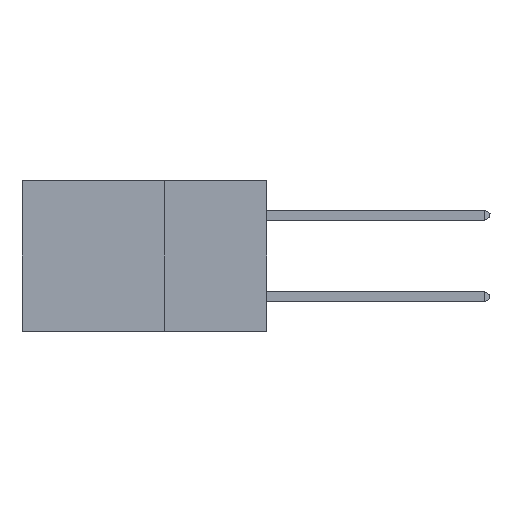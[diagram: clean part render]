
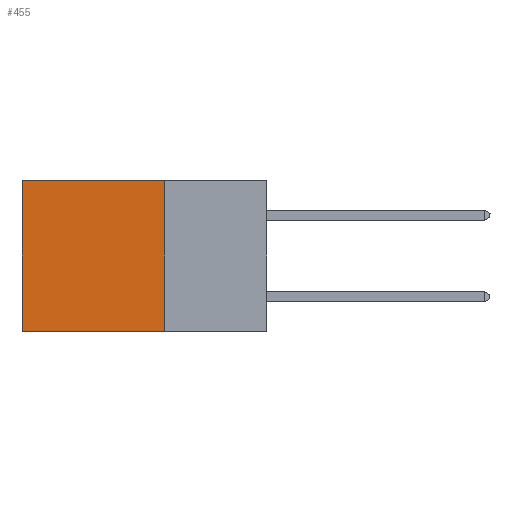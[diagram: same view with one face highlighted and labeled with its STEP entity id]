
A CAD part, left-side view. The second image highlights one B-rep face of the part: STEP entity #455.
In plain terms, the highlighted planar face has unit normal (-1, 0, 0).
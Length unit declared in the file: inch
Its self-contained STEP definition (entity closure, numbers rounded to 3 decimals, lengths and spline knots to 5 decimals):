
#174 = AXIS2_PLACEMENT_3D ( 'NONE', #11066, #1881, #10893 ) ;
#455 = ADVANCED_FACE ( 'NONE', ( #9174 ), #5852, .F. ) ;
#1270 = ORIENTED_EDGE ( 'NONE', *, *, #15241, .T. ) ;
#1368 = ORIENTED_EDGE ( 'NONE', *, *, #4803, .F. ) ;
#1848 = CARTESIAN_POINT ( 'NONE',  ( 0.2875, 0.25, 0. ) ) ;
#1881 = DIRECTION ( 'NONE',  ( 1., 0., 0. ) ) ;
#2020 = VERTEX_POINT ( 'NONE', #3974 ) ;
#2173 = ORIENTED_EDGE ( 'NONE', *, *, #13967, .T. ) ;
#3348 = VECTOR ( 'NONE', #14792, 39.37008 ) ;
#3591 = VECTOR ( 'NONE', #13160, 39.37008 ) ;
#3739 = CARTESIAN_POINT ( 'NONE',  ( 0.2875, 0.6, 0. ) ) ;
#3864 = CARTESIAN_POINT ( 'NONE',  ( 0.2875, 0.25, -0.37 ) ) ;
#3974 = CARTESIAN_POINT ( 'NONE',  ( 0.2875, 0.25, -0.37 ) ) ;
#4043 = CARTESIAN_POINT ( 'NONE',  ( 0.2875, 0.25, 0. ) ) ;
#4803 = EDGE_CURVE ( 'NONE', #2020, #5344, #15485, .T. ) ;
#4943 = VECTOR ( 'NONE', #8855, 39.37008 ) ;
#5191 = CARTESIAN_POINT ( 'NONE',  ( 0.2875, 0.25, 0. ) ) ;
#5344 = VERTEX_POINT ( 'NONE', #14591 ) ;
#5852 = PLANE ( 'NONE',  #174 ) ;
#6824 = LINE ( 'NONE', #4043, #3591 ) ;
#7399 = CARTESIAN_POINT ( 'NONE',  ( 0.2875, 0.6, 0. ) ) ;
#7976 = VECTOR ( 'NONE', #14007, 39.37008 ) ;
#8301 = VERTEX_POINT ( 'NONE', #5191 ) ;
#8637 = EDGE_LOOP ( 'NONE', ( #1270, #1368, #16489, #2173 ) ) ;
#8855 = DIRECTION ( 'NONE',  ( 0., 1., 0. ) ) ;
#9174 = FACE_OUTER_BOUND ( 'NONE', #8637, .T. ) ;
#9202 = VERTEX_POINT ( 'NONE', #3739 ) ;
#10893 = DIRECTION ( 'NONE',  ( 0., 0., -1. ) ) ;
#11066 = CARTESIAN_POINT ( 'NONE',  ( 0.2875, 0.25, 0. ) ) ;
#13160 = DIRECTION ( 'NONE',  ( 0., 1., 0. ) ) ;
#13265 = LINE ( 'NONE', #1848, #3348 ) ;
#13467 = LINE ( 'NONE', #7399, #7976 ) ;
#13967 = EDGE_CURVE ( 'NONE', #8301, #9202, #6824, .T. ) ;
#14007 = DIRECTION ( 'NONE',  ( 0., 0., -1. ) ) ;
#14591 = CARTESIAN_POINT ( 'NONE',  ( 0.2875, 0.6, -0.37 ) ) ;
#14775 = EDGE_CURVE ( 'NONE', #8301, #2020, #13265, .T. ) ;
#14792 = DIRECTION ( 'NONE',  ( 0., 0., -1. ) ) ;
#15241 = EDGE_CURVE ( 'NONE', #9202, #5344, #13467, .T. ) ;
#15485 = LINE ( 'NONE', #3864, #4943 ) ;
#16489 = ORIENTED_EDGE ( 'NONE', *, *, #14775, .F. ) ;
